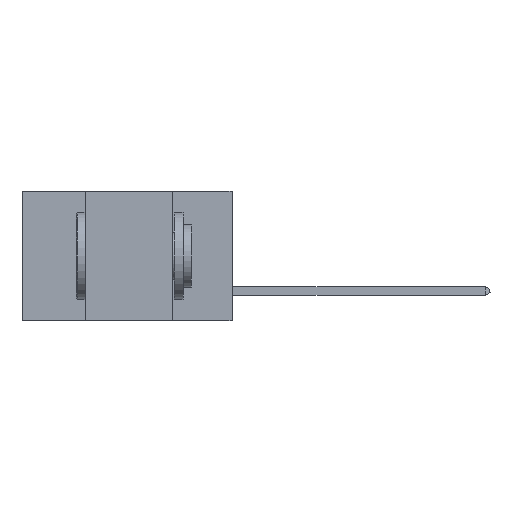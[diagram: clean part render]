
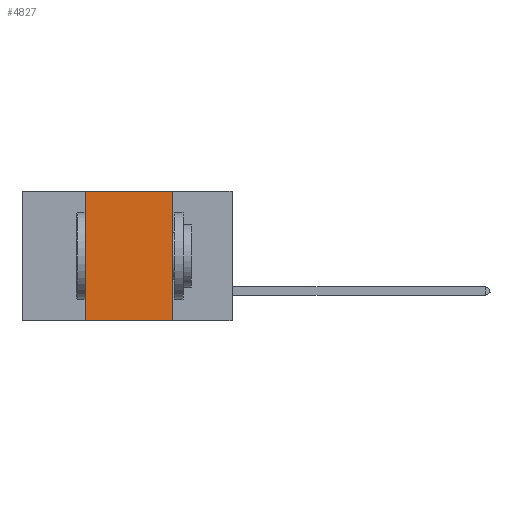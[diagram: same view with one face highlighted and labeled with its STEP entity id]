
A CAD part, left-side view. The second image highlights one B-rep face of the part: STEP entity #4827.
In plain terms, the highlighted planar face has unit normal (-1, 0, 0).
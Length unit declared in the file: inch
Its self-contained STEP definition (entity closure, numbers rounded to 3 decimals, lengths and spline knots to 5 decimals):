
#1020 = EDGE_CURVE ( 'NONE', #22030, #20898, #5845, .T. ) ;
#4207 = DIRECTION ( 'NONE',  ( 0., -1., 0. ) ) ;
#4423 = VECTOR ( 'NONE', #22470, 39.37008 ) ;
#4455 = EDGE_CURVE ( 'NONE', #18372, #6218, #10143, .T. ) ;
#4767 = DIRECTION ( 'NONE',  ( 0., 0., -1. ) ) ;
#4827 = ADVANCED_FACE ( 'NONE', ( #6945 ), #20833, .F. ) ;
#5492 = DIRECTION ( 'NONE',  ( 0., 0., 1. ) ) ;
#5845 = LINE ( 'NONE', #7771, #9902 ) ;
#5868 = ORIENTED_EDGE ( 'NONE', *, *, #20064, .F. ) ;
#6218 = VERTEX_POINT ( 'NONE', #10569 ) ;
#6945 = FACE_OUTER_BOUND ( 'NONE', #23598, .T. ) ;
#7771 = CARTESIAN_POINT ( 'NONE',  ( 0., 0.6, 0. ) ) ;
#8078 = DIRECTION ( 'NONE',  ( 0., -1., 0. ) ) ;
#9659 = CARTESIAN_POINT ( 'NONE',  ( 0., 0.17, 0. ) ) ;
#9902 = VECTOR ( 'NONE', #4207, 39.37008 ) ;
#10143 = LINE ( 'NONE', #13712, #19626 ) ;
#10569 = CARTESIAN_POINT ( 'NONE',  ( 0., 0.17, -0.37 ) ) ;
#10618 = CARTESIAN_POINT ( 'NONE',  ( 0., 0.42, 0. ) ) ;
#12625 = LINE ( 'NONE', #21624, #16375 ) ;
#12708 = ORIENTED_EDGE ( 'NONE', *, *, #4455, .T. ) ;
#13712 = CARTESIAN_POINT ( 'NONE',  ( 0., 0.6, -0.37 ) ) ;
#14188 = DIRECTION ( 'NONE',  ( 1., 0., 0. ) ) ;
#15430 = CARTESIAN_POINT ( 'NONE',  ( 0., 0.17, 0. ) ) ;
#15957 = ORIENTED_EDGE ( 'NONE', *, *, #1020, .F. ) ;
#16373 = EDGE_CURVE ( 'NONE', #20898, #6218, #18824, .T. ) ;
#16375 = VECTOR ( 'NONE', #5492, 39.37008 ) ;
#17646 = CARTESIAN_POINT ( 'NONE',  ( 0., 0.6, 0. ) ) ;
#18285 = ORIENTED_EDGE ( 'NONE', *, *, #16373, .F. ) ;
#18372 = VERTEX_POINT ( 'NONE', #19726 ) ;
#18824 = LINE ( 'NONE', #9659, #4423 ) ;
#19626 = VECTOR ( 'NONE', #8078, 39.37008 ) ;
#19726 = CARTESIAN_POINT ( 'NONE',  ( 0., 0.42, -0.37 ) ) ;
#20064 = EDGE_CURVE ( 'NONE', #18372, #22030, #12625, .T. ) ;
#20833 = PLANE ( 'NONE',  #22705 ) ;
#20898 = VERTEX_POINT ( 'NONE', #15430 ) ;
#21624 = CARTESIAN_POINT ( 'NONE',  ( 0., 0.42, 0. ) ) ;
#22030 = VERTEX_POINT ( 'NONE', #10618 ) ;
#22470 = DIRECTION ( 'NONE',  ( 0., 0., -1. ) ) ;
#22705 = AXIS2_PLACEMENT_3D ( 'NONE', #17646, #14188, #4767 ) ;
#23598 = EDGE_LOOP ( 'NONE', ( #18285, #15957, #5868, #12708 ) ) ;
